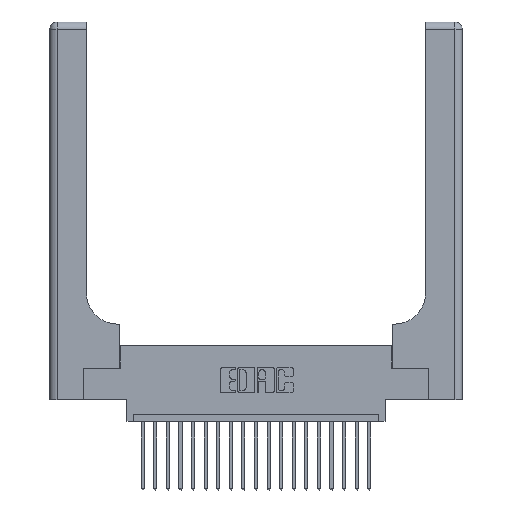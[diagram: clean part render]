
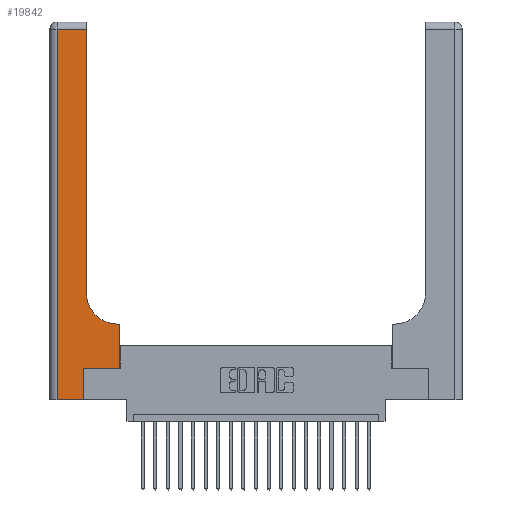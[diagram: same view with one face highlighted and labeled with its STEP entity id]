
A CAD part, top view. The second image highlights one B-rep face of the part: STEP entity #19842.
In plain terms, the highlighted planar face has unit normal (0, 0, 1).
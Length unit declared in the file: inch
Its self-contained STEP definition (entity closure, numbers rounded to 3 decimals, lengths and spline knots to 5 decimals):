
#74 = EDGE_CURVE ( 'NONE', #18560, #7362, #1601, .T. ) ;
#536 = EDGE_CURVE ( 'NONE', #14870, #570, #10872, .T. ) ;
#570 = VERTEX_POINT ( 'NONE', #7003 ) ;
#1560 = CARTESIAN_POINT ( 'NONE',  ( 0., 3., 0.37 ) ) ;
#1601 = LINE ( 'NONE', #7562, #2975 ) ;
#1644 = DIRECTION ( 'NONE',  ( 1., 0., 0. ) ) ;
#1785 = PLANE ( 'NONE',  #21450 ) ;
#1842 = VERTEX_POINT ( 'NONE', #10664 ) ;
#1995 = VECTOR ( 'NONE', #4161, 39.37008 ) ;
#2105 = VECTOR ( 'NONE', #20385, 39.37008 ) ;
#2946 = DIRECTION ( 'NONE',  ( -1., 0., 0. ) ) ;
#2975 = VECTOR ( 'NONE', #4159, 39.37008 ) ;
#3255 = VERTEX_POINT ( 'NONE', #9978 ) ;
#3379 = CARTESIAN_POINT ( 'NONE',  ( 0., 0., 0.37 ) ) ;
#4159 = DIRECTION ( 'NONE',  ( 0., 1., 0. ) ) ;
#4161 = DIRECTION ( 'NONE',  ( 0., 1., 0. ) ) ;
#4311 = CARTESIAN_POINT ( 'NONE',  ( 0.2915, 3., 0.37 ) ) ;
#5235 = EDGE_CURVE ( 'NONE', #1842, #14870, #13367, .T. ) ;
#6095 = LINE ( 'NONE', #4311, #1995 ) ;
#7003 = CARTESIAN_POINT ( 'NONE',  ( 0.269, 0., 0.37 ) ) ;
#7282 = LINE ( 'NONE', #14903, #2105 ) ;
#7362 = VERTEX_POINT ( 'NONE', #15218 ) ;
#7562 = CARTESIAN_POINT ( 'NONE',  ( 0.5585, 0.25, 0.37 ) ) ;
#7725 = CARTESIAN_POINT ( 'NONE',  ( 0.2915, 0.6, 0.37 ) ) ;
#7774 = ORIENTED_EDGE ( 'NONE', *, *, #15465, .T. ) ;
#8118 = DIRECTION ( 'NONE',  ( 0., -1., 0. ) ) ;
#9618 = CARTESIAN_POINT ( 'NONE',  ( 0.269, 0., 0.37 ) ) ;
#9757 = VECTOR ( 'NONE', #15053, 39.37008 ) ;
#9978 = CARTESIAN_POINT ( 'NONE',  ( 0.2915, 2.94, 0.37 ) ) ;
#9990 = CARTESIAN_POINT ( 'NONE',  ( 0.269, 0.25, 0.37 ) ) ;
#10266 = CARTESIAN_POINT ( 'NONE',  ( 0.5415, 0.6, 0.37 ) ) ;
#10664 = CARTESIAN_POINT ( 'NONE',  ( 0.06, 2.94, 0.37 ) ) ;
#10860 = LINE ( 'NONE', #9618, #9757 ) ;
#10872 = LINE ( 'NONE', #3379, #22143 ) ;
#10889 = ORIENTED_EDGE ( 'NONE', *, *, #13483, .T. ) ;
#10996 = CARTESIAN_POINT ( 'NONE',  ( 0.06, 0., 0.37 ) ) ;
#12252 = VECTOR ( 'NONE', #2946, 39.37008 ) ;
#12366 = CARTESIAN_POINT ( 'NONE',  ( 0.2915, 0.85, 0.37 ) ) ;
#12684 = DIRECTION ( 'NONE',  ( -1., 0., 0. ) ) ;
#12828 = CARTESIAN_POINT ( 'NONE',  ( 0., 2.94, 0.37 ) ) ;
#12971 = ORIENTED_EDGE ( 'NONE', *, *, #21522, .T. ) ;
#13367 = LINE ( 'NONE', #18653, #16153 ) ;
#13483 = EDGE_CURVE ( 'NONE', #21003, #3255, #6095, .T. ) ;
#13613 = DIRECTION ( 'NONE',  ( 0., 0., -1. ) ) ;
#14004 = DIRECTION ( 'NONE',  ( -1., 0., 0. ) ) ;
#14077 = DIRECTION ( 'NONE',  ( 0., 0., -1. ) ) ;
#14188 = ORIENTED_EDGE ( 'NONE', *, *, #16808, .T. ) ;
#14381 = AXIS2_PLACEMENT_3D ( 'NONE', #15497, #13613, #1644 ) ;
#14775 = VECTOR ( 'NONE', #12684, 39.37008 ) ;
#14817 = FACE_OUTER_BOUND ( 'NONE', #15388, .T. ) ;
#14870 = VERTEX_POINT ( 'NONE', #10996 ) ;
#14903 = CARTESIAN_POINT ( 'NONE',  ( 0.269, 0.25, 0.37 ) ) ;
#15053 = DIRECTION ( 'NONE',  ( 0., 1., 0. ) ) ;
#15218 = CARTESIAN_POINT ( 'NONE',  ( 0.5585, 0.6, 0.37 ) ) ;
#15311 = CARTESIAN_POINT ( 'NONE',  ( 0.5585, 0.25, 0.37 ) ) ;
#15388 = EDGE_LOOP ( 'NONE', ( #10889, #7774, #21405, #15740, #20354, #18251, #18676, #14188, #12971 ) ) ;
#15465 = EDGE_CURVE ( 'NONE', #3255, #1842, #19451, .T. ) ;
#15497 = CARTESIAN_POINT ( 'NONE',  ( 0.5415, 0.85, 0.37 ) ) ;
#15740 = ORIENTED_EDGE ( 'NONE', *, *, #536, .T. ) ;
#16153 = VECTOR ( 'NONE', #8118, 39.37008 ) ;
#16808 = EDGE_CURVE ( 'NONE', #7362, #16971, #17186, .T. ) ;
#16971 = VERTEX_POINT ( 'NONE', #10266 ) ;
#17186 = LINE ( 'NONE', #7725, #12252 ) ;
#18251 = ORIENTED_EDGE ( 'NONE', *, *, #21962, .T. ) ;
#18560 = VERTEX_POINT ( 'NONE', #15311 ) ;
#18653 = CARTESIAN_POINT ( 'NONE',  ( 0.06, 3., 0.37 ) ) ;
#18676 = ORIENTED_EDGE ( 'NONE', *, *, #74, .T. ) ;
#19451 = LINE ( 'NONE', #12828, #14775 ) ;
#19842 = ADVANCED_FACE ( 'NONE', ( #14817 ), #1785, .F. ) ;
#20354 = ORIENTED_EDGE ( 'NONE', *, *, #21929, .T. ) ;
#20385 = DIRECTION ( 'NONE',  ( 1., 0., 0. ) ) ;
#21003 = VERTEX_POINT ( 'NONE', #12366 ) ;
#21148 = DIRECTION ( 'NONE',  ( 1., 0., 0. ) ) ;
#21328 = CIRCLE ( 'NONE', #14381, 0.25 ) ;
#21405 = ORIENTED_EDGE ( 'NONE', *, *, #5235, .T. ) ;
#21450 = AXIS2_PLACEMENT_3D ( 'NONE', #1560, #14077, #14004 ) ;
#21522 = EDGE_CURVE ( 'NONE', #16971, #21003, #21328, .T. ) ;
#21929 = EDGE_CURVE ( 'NONE', #570, #22076, #10860, .T. ) ;
#21962 = EDGE_CURVE ( 'NONE', #22076, #18560, #7282, .T. ) ;
#22076 = VERTEX_POINT ( 'NONE', #9990 ) ;
#22143 = VECTOR ( 'NONE', #21148, 39.37008 ) ;
